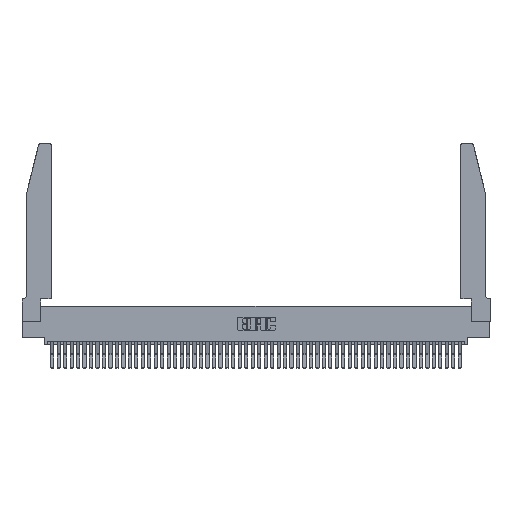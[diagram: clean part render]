
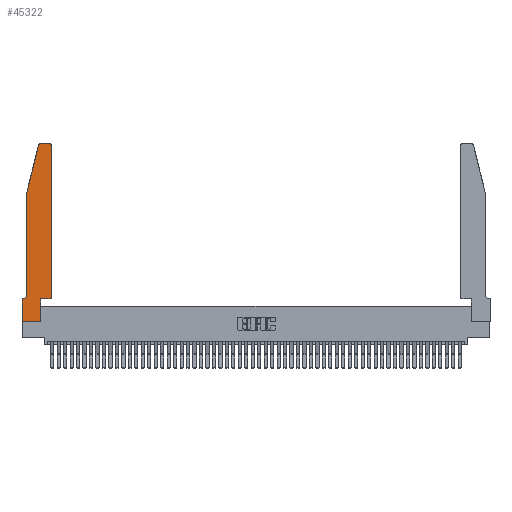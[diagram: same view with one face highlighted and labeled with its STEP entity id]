
A CAD part, top view. The second image highlights one B-rep face of the part: STEP entity #45322.
In plain terms, the highlighted planar face has unit normal (0, 0, 1).
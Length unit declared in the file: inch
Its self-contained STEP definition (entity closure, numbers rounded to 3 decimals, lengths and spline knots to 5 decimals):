
#182 = CIRCLE ( 'NONE', #12392, 0.07 ) ;
#659 = LINE ( 'NONE', #20534, #49950 ) ;
#661 = DIRECTION ( 'NONE',  ( 0., -1., 0. ) ) ;
#1274 = EDGE_CURVE ( 'NONE', #42974, #45809, #14176, .T. ) ;
#2076 = CARTESIAN_POINT ( 'NONE',  ( 0.0755, 0.42, 0.37 ) ) ;
#2432 = CIRCLE ( 'NONE', #28244, 0.03 ) ;
#2490 = EDGE_CURVE ( 'NONE', #48819, #7559, #45627, .T. ) ;
#2793 = VECTOR ( 'NONE', #20782, 39.37008 ) ;
#3193 = EDGE_CURVE ( 'NONE', #26988, #48759, #24101, .T. ) ;
#3223 = ORIENTED_EDGE ( 'NONE', *, *, #18326, .T. ) ;
#3559 = VECTOR ( 'NONE', #13257, 39.37008 ) ;
#3670 = CARTESIAN_POINT ( 'NONE',  ( 0.284, 2.72, 0.37 ) ) ;
#3911 = LINE ( 'NONE', #34001, #45600 ) ;
#4664 = DIRECTION ( 'NONE',  ( -0.239, -0.971, 0. ) ) ;
#4730 = DIRECTION ( 'NONE',  ( 0., 0., -1. ) ) ;
#5641 = DIRECTION ( 'NONE',  ( 1., 0., 0. ) ) ;
#6550 = CARTESIAN_POINT ( 'NONE',  ( 0.4505, 0.35, 0.37 ) ) ;
#6860 = DIRECTION ( 'NONE',  ( 0., 0., 1. ) ) ;
#6982 = DIRECTION ( 'NONE',  ( 1., 0., 0. ) ) ;
#7559 = VERTEX_POINT ( 'NONE', #32617 ) ;
#8125 = ORIENTED_EDGE ( 'NONE', *, *, #14282, .T. ) ;
#9113 = DIRECTION ( 'NONE',  ( -1., 0., 0. ) ) ;
#10568 = ORIENTED_EDGE ( 'NONE', *, *, #42738, .T. ) ;
#10777 = DIRECTION ( 'NONE',  ( 1., 0., 0. ) ) ;
#11097 = CARTESIAN_POINT ( 'NONE',  ( 0.4505, 0.35, 0.37 ) ) ;
#11152 = LINE ( 'NONE', #6550, #24994 ) ;
#11521 = VECTOR ( 'NONE', #16991, 39.37008 ) ;
#12392 = AXIS2_PLACEMENT_3D ( 'NONE', #33299, #4730, #9113 ) ;
#12485 = ORIENTED_EDGE ( 'NONE', *, *, #2490, .T. ) ;
#12591 = VECTOR ( 'NONE', #43107, 39.37008 ) ;
#12997 = EDGE_CURVE ( 'NONE', #7559, #33946, #50602, .T. ) ;
#13160 = CARTESIAN_POINT ( 'NONE',  ( 0.4505, 2.72, 0.37 ) ) ;
#13257 = DIRECTION ( 'NONE',  ( 0., 1., 0. ) ) ;
#13527 = DIRECTION ( 'NONE',  ( 0., 1., 0. ) ) ;
#13867 = ORIENTED_EDGE ( 'NONE', *, *, #29754, .T. ) ;
#14176 = LINE ( 'NONE', #33137, #2793 ) ;
#14282 = EDGE_CURVE ( 'NONE', #45787, #51490, #21458, .T. ) ;
#15083 = CARTESIAN_POINT ( 'NONE',  ( 0.4205, 2.75, 0.37 ) ) ;
#15969 = AXIS2_PLACEMENT_3D ( 'NONE', #3670, #6860, #31238 ) ;
#16571 = ORIENTED_EDGE ( 'NONE', *, *, #43504, .T. ) ;
#16687 = CARTESIAN_POINT ( 'NONE',  ( 0.2605, 2.75, 0.37 ) ) ;
#16841 = FACE_OUTER_BOUND ( 'NONE', #21096, .T. ) ;
#16991 = DIRECTION ( 'NONE',  ( 0., -1., 0. ) ) ;
#17361 = CARTESIAN_POINT ( 'NONE',  ( 0.2865, 0., 0.37 ) ) ;
#17708 = CARTESIAN_POINT ( 'NONE',  ( 0.0055, 0.35, 0.37 ) ) ;
#18326 = EDGE_CURVE ( 'NONE', #41184, #48819, #2432, .T. ) ;
#20534 = CARTESIAN_POINT ( 'NONE',  ( 0.0755, 2., 0.37 ) ) ;
#20782 = DIRECTION ( 'NONE',  ( 1., 0., 0. ) ) ;
#21096 = EDGE_LOOP ( 'NONE', ( #12485, #23068, #16571, #38060, #33361, #8125, #10568, #46721, #13867, #41219, #24397, #3223 ) ) ;
#21458 = LINE ( 'NONE', #30966, #12591 ) ;
#21683 = DIRECTION ( 'NONE',  ( 0., 0., 1. ) ) ;
#23068 = ORIENTED_EDGE ( 'NONE', *, *, #12997, .T. ) ;
#23496 = AXIS2_PLACEMENT_3D ( 'NONE', #30839, #42985, #6982 ) ;
#24101 = LINE ( 'NONE', #40985, #11521 ) ;
#24397 = ORIENTED_EDGE ( 'NONE', *, *, #32979, .T. ) ;
#24994 = VECTOR ( 'NONE', #10777, 39.37008 ) ;
#25619 = CARTESIAN_POINT ( 'NONE',  ( 0.2865, 0.35, 0.37 ) ) ;
#26988 = VERTEX_POINT ( 'NONE', #28441 ) ;
#28244 = AXIS2_PLACEMENT_3D ( 'NONE', #41628, #21683, #5641 ) ;
#28441 = CARTESIAN_POINT ( 'NONE',  ( 0.0755, 2., 0.37 ) ) ;
#28553 = VECTOR ( 'NONE', #49199, 39.37008 ) ;
#29754 = EDGE_CURVE ( 'NONE', #45809, #30804, #40809, .T. ) ;
#29917 = EDGE_CURVE ( 'NONE', #30804, #42564, #11152, .T. ) ;
#30451 = LINE ( 'NONE', #41048, #33572 ) ;
#30804 = VERTEX_POINT ( 'NONE', #31387 ) ;
#30839 = CARTESIAN_POINT ( 'NONE',  ( 0., 0.35, 0.37 ) ) ;
#30966 = CARTESIAN_POINT ( 'NONE',  ( 0.0755, 0.35, 0.37 ) ) ;
#31238 = DIRECTION ( 'NONE',  ( 1., 0., 0. ) ) ;
#31387 = CARTESIAN_POINT ( 'NONE',  ( 0.2865, 0.35, 0.37 ) ) ;
#32617 = CARTESIAN_POINT ( 'NONE',  ( 0.284, 2.75, 0.37 ) ) ;
#32753 = EDGE_CURVE ( 'NONE', #48759, #45787, #182, .T. ) ;
#32979 = EDGE_CURVE ( 'NONE', #42564, #41184, #3911, .T. ) ;
#33137 = CARTESIAN_POINT ( 'NONE',  ( 0., 0., 0.37 ) ) ;
#33299 = CARTESIAN_POINT ( 'NONE',  ( 0.0055, 0.42, 0.37 ) ) ;
#33361 = ORIENTED_EDGE ( 'NONE', *, *, #32753, .T. ) ;
#33572 = VECTOR ( 'NONE', #661, 39.37008 ) ;
#33946 = VERTEX_POINT ( 'NONE', #44120 ) ;
#33997 = CARTESIAN_POINT ( 'NONE',  ( 0., 0., 0.37 ) ) ;
#34001 = CARTESIAN_POINT ( 'NONE',  ( 0.4505, 0.35, 0.37 ) ) ;
#38060 = ORIENTED_EDGE ( 'NONE', *, *, #3193, .T. ) ;
#40809 = LINE ( 'NONE', #25619, #3559 ) ;
#40985 = CARTESIAN_POINT ( 'NONE',  ( 0.0755, 2., 0.37 ) ) ;
#41021 = CARTESIAN_POINT ( 'NONE',  ( 0., 0.35, 0.37 ) ) ;
#41048 = CARTESIAN_POINT ( 'NONE',  ( 0., 0., 0.37 ) ) ;
#41184 = VERTEX_POINT ( 'NONE', #13160 ) ;
#41219 = ORIENTED_EDGE ( 'NONE', *, *, #29917, .T. ) ;
#41628 = CARTESIAN_POINT ( 'NONE',  ( 0.4205, 2.72, 0.37 ) ) ;
#42564 = VERTEX_POINT ( 'NONE', #11097 ) ;
#42738 = EDGE_CURVE ( 'NONE', #51490, #42974, #30451, .T. ) ;
#42974 = VERTEX_POINT ( 'NONE', #33997 ) ;
#42985 = DIRECTION ( 'NONE',  ( 0., 0., 1. ) ) ;
#43107 = DIRECTION ( 'NONE',  ( -1., 0., 0. ) ) ;
#43168 = PLANE ( 'NONE',  #23496 ) ;
#43504 = EDGE_CURVE ( 'NONE', #33946, #26988, #659, .T. ) ;
#44120 = CARTESIAN_POINT ( 'NONE',  ( 0.25487, 2.72718, 0.37 ) ) ;
#45322 = ADVANCED_FACE ( 'NONE', ( #16841 ), #43168, .T. ) ;
#45600 = VECTOR ( 'NONE', #13527, 39.37008 ) ;
#45627 = LINE ( 'NONE', #16687, #28553 ) ;
#45787 = VERTEX_POINT ( 'NONE', #17708 ) ;
#45809 = VERTEX_POINT ( 'NONE', #17361 ) ;
#46721 = ORIENTED_EDGE ( 'NONE', *, *, #1274, .T. ) ;
#48759 = VERTEX_POINT ( 'NONE', #2076 ) ;
#48819 = VERTEX_POINT ( 'NONE', #15083 ) ;
#49199 = DIRECTION ( 'NONE',  ( -1., 0., 0. ) ) ;
#49950 = VECTOR ( 'NONE', #4664, 39.37008 ) ;
#50602 = CIRCLE ( 'NONE', #15969, 0.03 ) ;
#51490 = VERTEX_POINT ( 'NONE', #41021 ) ;
